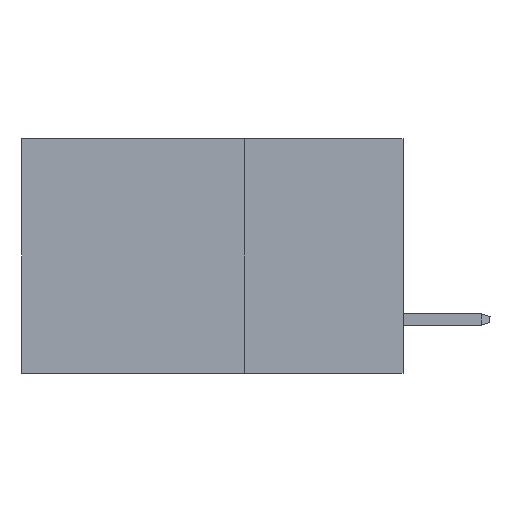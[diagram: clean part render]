
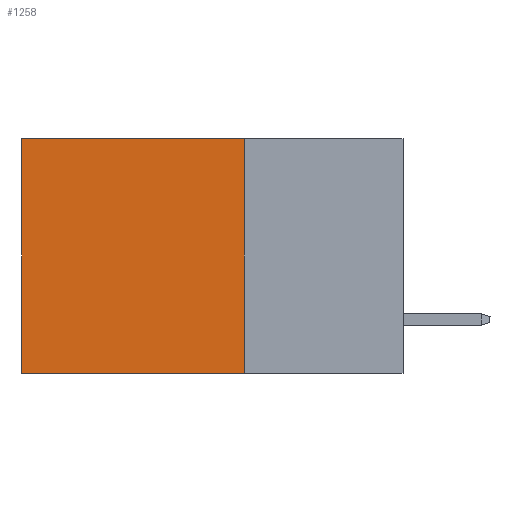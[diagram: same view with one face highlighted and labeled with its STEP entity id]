
A CAD part, left-side view. The second image highlights one B-rep face of the part: STEP entity #1258.
In plain terms, the highlighted planar face has unit normal (-1, 0, 0).
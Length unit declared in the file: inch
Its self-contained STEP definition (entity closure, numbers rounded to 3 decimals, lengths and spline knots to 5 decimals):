
#1258 = ADVANCED_FACE ( 'NONE', ( #13001 ), #22100, .F. ) ;
#1841 = CARTESIAN_POINT ( 'NONE',  ( 0.2875, 0.25, 0. ) ) ;
#2092 = CARTESIAN_POINT ( 'NONE',  ( 0.2875, 0.6, 0. ) ) ;
#2457 = ORIENTED_EDGE ( 'NONE', *, *, #8149, .F. ) ;
#3626 = EDGE_LOOP ( 'NONE', ( #15491, #2457, #14983, #26489 ) ) ;
#4230 = LINE ( 'NONE', #13039, #24085 ) ;
#4478 = CARTESIAN_POINT ( 'NONE',  ( 0.2875, 0.25, 0. ) ) ;
#5518 = VERTEX_POINT ( 'NONE', #9473 ) ;
#6316 = LINE ( 'NONE', #1841, #19072 ) ;
#8149 = EDGE_CURVE ( 'NONE', #5518, #15862, #22133, .T. ) ;
#8932 = DIRECTION ( 'NONE',  ( 0., 0., -1. ) ) ;
#9123 = CARTESIAN_POINT ( 'NONE',  ( 0.2875, 0.25, -0.37 ) ) ;
#9473 = CARTESIAN_POINT ( 'NONE',  ( 0.2875, 0.25, -0.37 ) ) ;
#11136 = DIRECTION ( 'NONE',  ( 0., 1., 0. ) ) ;
#11237 = CARTESIAN_POINT ( 'NONE',  ( 0.2875, 0.6, 0. ) ) ;
#12703 = VECTOR ( 'NONE', #21886, 39.37008 ) ;
#12998 = CARTESIAN_POINT ( 'NONE',  ( 0.2875, 0.25, 0. ) ) ;
#13001 = FACE_OUTER_BOUND ( 'NONE', #3626, .T. ) ;
#13039 = CARTESIAN_POINT ( 'NONE',  ( 0.2875, 0.25, 0. ) ) ;
#13186 = AXIS2_PLACEMENT_3D ( 'NONE', #4478, #17769, #8932 ) ;
#14966 = LINE ( 'NONE', #2092, #12703 ) ;
#14983 = ORIENTED_EDGE ( 'NONE', *, *, #18128, .F. ) ;
#15133 = CARTESIAN_POINT ( 'NONE',  ( 0.2875, 0.6, -0.37 ) ) ;
#15365 = VERTEX_POINT ( 'NONE', #12998 ) ;
#15491 = ORIENTED_EDGE ( 'NONE', *, *, #25765, .T. ) ;
#15862 = VERTEX_POINT ( 'NONE', #15133 ) ;
#17143 = EDGE_CURVE ( 'NONE', #15365, #28046, #6316, .T. ) ;
#17769 = DIRECTION ( 'NONE',  ( 1., 0., 0. ) ) ;
#18128 = EDGE_CURVE ( 'NONE', #15365, #5518, #4230, .T. ) ;
#19072 = VECTOR ( 'NONE', #21492, 39.37008 ) ;
#19160 = DIRECTION ( 'NONE',  ( 0., 0., -1. ) ) ;
#21492 = DIRECTION ( 'NONE',  ( 0., 1., 0. ) ) ;
#21886 = DIRECTION ( 'NONE',  ( 0., 0., -1. ) ) ;
#22100 = PLANE ( 'NONE',  #13186 ) ;
#22133 = LINE ( 'NONE', #9123, #27229 ) ;
#24085 = VECTOR ( 'NONE', #19160, 39.37008 ) ;
#25765 = EDGE_CURVE ( 'NONE', #28046, #15862, #14966, .T. ) ;
#26489 = ORIENTED_EDGE ( 'NONE', *, *, #17143, .T. ) ;
#27229 = VECTOR ( 'NONE', #11136, 39.37008 ) ;
#28046 = VERTEX_POINT ( 'NONE', #11237 ) ;
